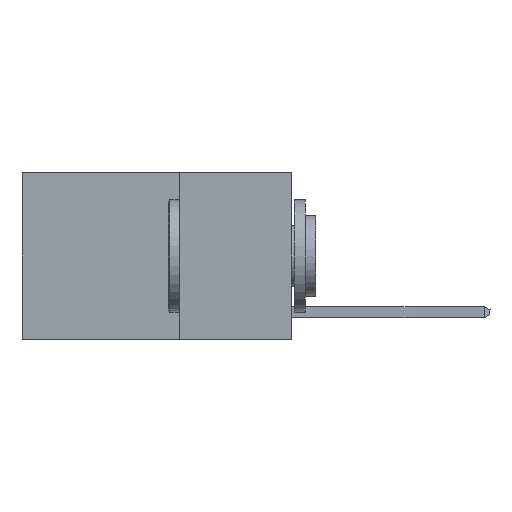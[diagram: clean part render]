
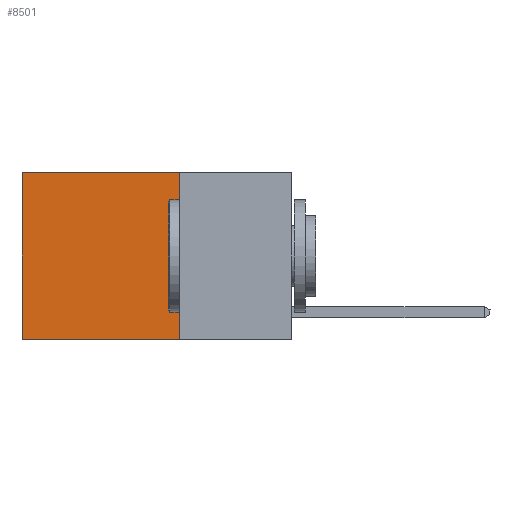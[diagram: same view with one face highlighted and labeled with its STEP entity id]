
A CAD part, left-side view. The second image highlights one B-rep face of the part: STEP entity #8501.
In plain terms, the highlighted planar face has unit normal (-1, 0, 0).
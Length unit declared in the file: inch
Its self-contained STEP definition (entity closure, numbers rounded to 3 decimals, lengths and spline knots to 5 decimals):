
#558 = FACE_OUTER_BOUND ( 'NONE', #7978, .T. ) ;
#830 = ORIENTED_EDGE ( 'NONE', *, *, #19308, .F. ) ;
#1922 = CARTESIAN_POINT ( 'NONE',  ( 0.2625, 0.25, 0. ) ) ;
#2152 = VERTEX_POINT ( 'NONE', #6670 ) ;
#2174 = LINE ( 'NONE', #1922, #5944 ) ;
#2514 = CARTESIAN_POINT ( 'NONE',  ( 0.2625, 0.25, -0.37 ) ) ;
#3556 = ORIENTED_EDGE ( 'NONE', *, *, #6522, .F. ) ;
#3763 = DIRECTION ( 'NONE',  ( 0., 0., -1. ) ) ;
#4951 = EDGE_CURVE ( 'NONE', #2152, #12315, #21849, .T. ) ;
#5353 = ORIENTED_EDGE ( 'NONE', *, *, #4951, .T. ) ;
#5944 = VECTOR ( 'NONE', #15226, 39.37008 ) ;
#6125 = CARTESIAN_POINT ( 'NONE',  ( 0.2625, 0.6, 0. ) ) ;
#6522 = EDGE_CURVE ( 'NONE', #19495, #7188, #9798, .T. ) ;
#6616 = CARTESIAN_POINT ( 'NONE',  ( 0.2625, 0.25, -0.37 ) ) ;
#6670 = CARTESIAN_POINT ( 'NONE',  ( 0.2625, 0.25, 0. ) ) ;
#7188 = VERTEX_POINT ( 'NONE', #23144 ) ;
#7312 = DIRECTION ( 'NONE',  ( 1., 0., 0. ) ) ;
#7488 = CARTESIAN_POINT ( 'NONE',  ( 0.2625, 0.25, 0. ) ) ;
#7978 = EDGE_LOOP ( 'NONE', ( #17106, #3556, #830, #5353 ) ) ;
#8079 = VECTOR ( 'NONE', #16498, 39.37008 ) ;
#8501 = ADVANCED_FACE ( 'NONE', ( #558 ), #22562, .F. ) ;
#9798 = LINE ( 'NONE', #2514, #15950 ) ;
#10973 = AXIS2_PLACEMENT_3D ( 'NONE', #7488, #7312, #3763 ) ;
#11755 = VECTOR ( 'NONE', #13329, 39.37008 ) ;
#12315 = VERTEX_POINT ( 'NONE', #6125 ) ;
#13053 = LINE ( 'NONE', #20342, #8079 ) ;
#13329 = DIRECTION ( 'NONE',  ( 0., 1., 0. ) ) ;
#15226 = DIRECTION ( 'NONE',  ( 0., 0., -1. ) ) ;
#15577 = DIRECTION ( 'NONE',  ( 0., 1., 0. ) ) ;
#15950 = VECTOR ( 'NONE', #15577, 39.37008 ) ;
#16498 = DIRECTION ( 'NONE',  ( 0., 0., -1. ) ) ;
#17106 = ORIENTED_EDGE ( 'NONE', *, *, #17615, .T. ) ;
#17615 = EDGE_CURVE ( 'NONE', #12315, #7188, #13053, .T. ) ;
#19308 = EDGE_CURVE ( 'NONE', #2152, #19495, #2174, .T. ) ;
#19495 = VERTEX_POINT ( 'NONE', #6616 ) ;
#20342 = CARTESIAN_POINT ( 'NONE',  ( 0.2625, 0.6, 0. ) ) ;
#20979 = CARTESIAN_POINT ( 'NONE',  ( 0.2625, 0.25, 0. ) ) ;
#21849 = LINE ( 'NONE', #20979, #11755 ) ;
#22562 = PLANE ( 'NONE',  #10973 ) ;
#23144 = CARTESIAN_POINT ( 'NONE',  ( 0.2625, 0.6, -0.37 ) ) ;
